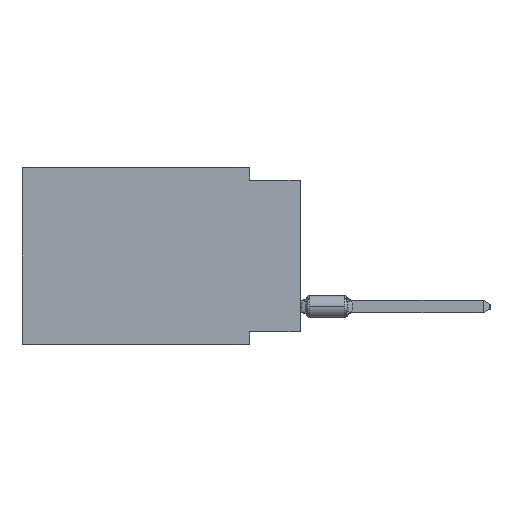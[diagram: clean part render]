
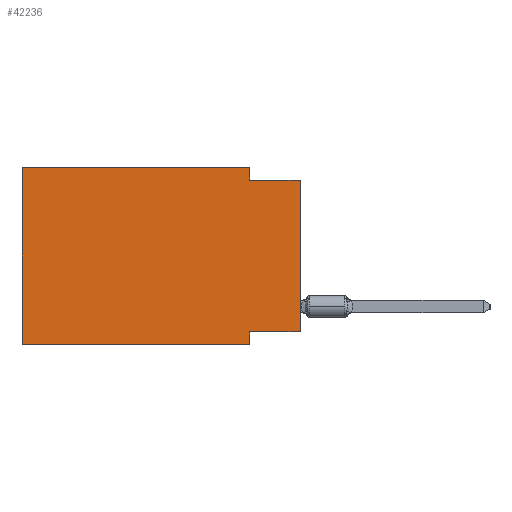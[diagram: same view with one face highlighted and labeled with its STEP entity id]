
A CAD part, left-side view. The second image highlights one B-rep face of the part: STEP entity #42236.
In plain terms, the highlighted planar face has unit normal (-1, 0, 0).
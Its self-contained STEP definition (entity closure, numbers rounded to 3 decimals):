
#294 = DIRECTION ( 'NONE',  ( 0., 0., -1. ) ) ;
#352 = CARTESIAN_POINT ( 'NONE',  ( 0., 0., -0.635 ) ) ;
#812 = DIRECTION ( 'NONE',  ( 0., -1., 0. ) ) ;
#1216 = AXIS2_PLACEMENT_3D ( 'NONE', #24181, #17559, #38995 ) ;
#1767 = EDGE_CURVE ( 'NONE', #11034, #36161, #15756, .T. ) ;
#1835 = CARTESIAN_POINT ( 'NONE',  ( 0., 2.54, 0. ) ) ;
#2038 = EDGE_CURVE ( 'NONE', #36496, #23079, #33087, .T. ) ;
#3846 = DIRECTION ( 'NONE',  ( 0., 0., 1. ) ) ;
#7006 = CARTESIAN_POINT ( 'NONE',  ( 0., 13.97, -8.89 ) ) ;
#7190 = CARTESIAN_POINT ( 'NONE',  ( 0., 0., -8.255 ) ) ;
#9150 = DIRECTION ( 'NONE',  ( 0., 1., 0. ) ) ;
#10327 = VECTOR ( 'NONE', #21837, 1000. ) ;
#11034 = VERTEX_POINT ( 'NONE', #7190 ) ;
#11223 = LINE ( 'NONE', #352, #10327 ) ;
#11292 = VECTOR ( 'NONE', #294, 1000. ) ;
#12438 = CARTESIAN_POINT ( 'NONE',  ( 0., 0., -8.255 ) ) ;
#14446 = ORIENTED_EDGE ( 'NONE', *, *, #22096, .F. ) ;
#14465 = LINE ( 'NONE', #32817, #33489 ) ;
#15662 = VECTOR ( 'NONE', #36612, 1000. ) ;
#15756 = LINE ( 'NONE', #12438, #31613 ) ;
#16296 = CARTESIAN_POINT ( 'NONE',  ( 0., 13.97, 0. ) ) ;
#16453 = ORIENTED_EDGE ( 'NONE', *, *, #39406, .F. ) ;
#16991 = DIRECTION ( 'NONE',  ( 0., 0., -1. ) ) ;
#17307 = VECTOR ( 'NONE', #16991, 1000. ) ;
#17518 = VERTEX_POINT ( 'NONE', #1835 ) ;
#17559 = DIRECTION ( 'NONE',  ( 1., 0., 0. ) ) ;
#17728 = ORIENTED_EDGE ( 'NONE', *, *, #43393, .F. ) ;
#17771 = CARTESIAN_POINT ( 'NONE',  ( 0., 2.54, -8.89 ) ) ;
#18290 = VERTEX_POINT ( 'NONE', #19184 ) ;
#18725 = CARTESIAN_POINT ( 'NONE',  ( 0., 13.97, -8.89 ) ) ;
#19184 = CARTESIAN_POINT ( 'NONE',  ( 0., 2.54, -0.635 ) ) ;
#20175 = FACE_OUTER_BOUND ( 'NONE', #42809, .T. ) ;
#20767 = LINE ( 'NONE', #38194, #17307 ) ;
#20894 = LINE ( 'NONE', #32806, #31649 ) ;
#21837 = DIRECTION ( 'NONE',  ( 0., -1., 0. ) ) ;
#22096 = EDGE_CURVE ( 'NONE', #26327, #17518, #34183, .T. ) ;
#22389 = ORIENTED_EDGE ( 'NONE', *, *, #42305, .F. ) ;
#23079 = VERTEX_POINT ( 'NONE', #32370 ) ;
#24029 = ORIENTED_EDGE ( 'NONE', *, *, #37148, .F. ) ;
#24181 = CARTESIAN_POINT ( 'NONE',  ( 0., 13.97, 0. ) ) ;
#25440 = CARTESIAN_POINT ( 'NONE',  ( 0., 2.54, -8.255 ) ) ;
#26327 = VERTEX_POINT ( 'NONE', #45490 ) ;
#26902 = VERTEX_POINT ( 'NONE', #29150 ) ;
#28178 = DIRECTION ( 'NONE',  ( 0., 0., 1. ) ) ;
#29150 = CARTESIAN_POINT ( 'NONE',  ( 0., 0., -0.635 ) ) ;
#31613 = VECTOR ( 'NONE', #9150, 1000. ) ;
#31649 = VECTOR ( 'NONE', #28178, 1000. ) ;
#31852 = EDGE_CURVE ( 'NONE', #11034, #26902, #14465, .T. ) ;
#32370 = CARTESIAN_POINT ( 'NONE',  ( 0., 2.54, -8.89 ) ) ;
#32806 = CARTESIAN_POINT ( 'NONE',  ( 0., 13.97, 0. ) ) ;
#32817 = CARTESIAN_POINT ( 'NONE',  ( 0., 0., 0. ) ) ;
#33087 = LINE ( 'NONE', #18725, #15662 ) ;
#33489 = VECTOR ( 'NONE', #3846, 1000. ) ;
#34183 = LINE ( 'NONE', #16296, #42495 ) ;
#34525 = PLANE ( 'NONE',  #1216 ) ;
#36130 = LINE ( 'NONE', #17771, #11292 ) ;
#36161 = VERTEX_POINT ( 'NONE', #25440 ) ;
#36496 = VERTEX_POINT ( 'NONE', #7006 ) ;
#36612 = DIRECTION ( 'NONE',  ( 0., -1., 0. ) ) ;
#37148 = EDGE_CURVE ( 'NONE', #17518, #18290, #20767, .T. ) ;
#38194 = CARTESIAN_POINT ( 'NONE',  ( 0., 2.54, 0. ) ) ;
#38995 = DIRECTION ( 'NONE',  ( 0., 0., -1. ) ) ;
#39406 = EDGE_CURVE ( 'NONE', #36161, #23079, #36130, .T. ) ;
#40610 = ORIENTED_EDGE ( 'NONE', *, *, #31852, .T. ) ;
#42236 = ADVANCED_FACE ( 'NONE', ( #20175 ), #34525, .F. ) ;
#42305 = EDGE_CURVE ( 'NONE', #36496, #26327, #20894, .T. ) ;
#42495 = VECTOR ( 'NONE', #812, 1000. ) ;
#42809 = EDGE_LOOP ( 'NONE', ( #40610, #17728, #24029, #14446, #22389, #46484, #16453, #43186 ) ) ;
#43186 = ORIENTED_EDGE ( 'NONE', *, *, #1767, .F. ) ;
#43393 = EDGE_CURVE ( 'NONE', #18290, #26902, #11223, .T. ) ;
#45490 = CARTESIAN_POINT ( 'NONE',  ( 0., 13.97, 0. ) ) ;
#46484 = ORIENTED_EDGE ( 'NONE', *, *, #2038, .T. ) ;
